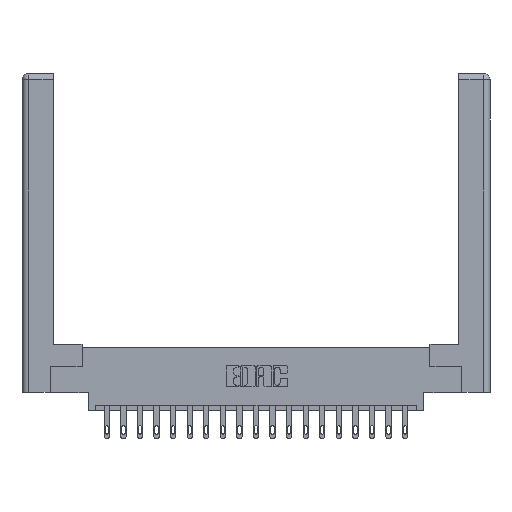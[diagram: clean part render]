
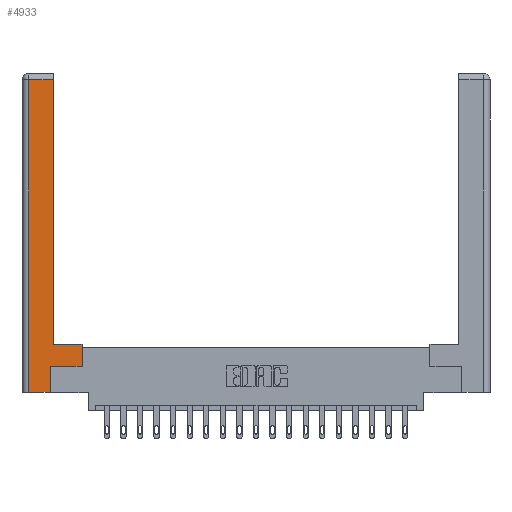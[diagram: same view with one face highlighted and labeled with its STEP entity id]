
A CAD part, top view. The second image highlights one B-rep face of the part: STEP entity #4933.
In plain terms, the highlighted planar face has unit normal (0, 0, 1).
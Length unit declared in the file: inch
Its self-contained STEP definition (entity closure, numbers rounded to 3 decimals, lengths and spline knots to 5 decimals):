
#195 = ORIENTED_EDGE ( 'NONE', *, *, #1138, .T. ) ;
#403 = VECTOR ( 'NONE', #12427, 39.37008 ) ;
#427 = LINE ( 'NONE', #4346, #16704 ) ;
#886 = LINE ( 'NONE', #3067, #8757 ) ;
#923 = DIRECTION ( 'NONE',  ( 1., 0., 0. ) ) ;
#1138 = EDGE_CURVE ( 'NONE', #15980, #16227, #7756, .T. ) ;
#1324 = LINE ( 'NONE', #5678, #8692 ) ;
#1429 = CARTESIAN_POINT ( 'NONE',  ( 0.295, 0.45, 0. ) ) ;
#2410 = CARTESIAN_POINT ( 'NONE',  ( 0.295, 2.94, 0. ) ) ;
#2630 = DIRECTION ( 'NONE',  ( -1., 0., 0. ) ) ;
#2715 = VERTEX_POINT ( 'NONE', #19667 ) ;
#2999 = CARTESIAN_POINT ( 'NONE',  ( 0.565, 0.245, 0. ) ) ;
#3067 = CARTESIAN_POINT ( 'NONE',  ( 0.565, 0.45, 0. ) ) ;
#3170 = CARTESIAN_POINT ( 'NONE',  ( 0.265, 0.245, 0. ) ) ;
#3243 = ORIENTED_EDGE ( 'NONE', *, *, #6716, .T. ) ;
#3328 = VECTOR ( 'NONE', #16255, 39.37008 ) ;
#4346 = CARTESIAN_POINT ( 'NONE',  ( 0.295, 0.45, 0. ) ) ;
#4414 = CARTESIAN_POINT ( 'NONE',  ( 0.565, 0.245, 0. ) ) ;
#4787 = DIRECTION ( 'NONE',  ( 0., 1., 0. ) ) ;
#4933 = ADVANCED_FACE ( 'NONE', ( #6801 ), #9155, .F. ) ;
#5036 = VERTEX_POINT ( 'NONE', #4414 ) ;
#5079 = CARTESIAN_POINT ( 'NONE',  ( 0.0615, 2.94, 0. ) ) ;
#5248 = ORIENTED_EDGE ( 'NONE', *, *, #15515, .T. ) ;
#5678 = CARTESIAN_POINT ( 'NONE',  ( 0.265, 0., 0. ) ) ;
#5732 = CARTESIAN_POINT ( 'NONE',  ( 0.565, 0.45, 0. ) ) ;
#5932 = CARTESIAN_POINT ( 'NONE',  ( 0., 0., 0. ) ) ;
#6716 = EDGE_CURVE ( 'NONE', #18542, #18761, #1324, .T. ) ;
#6801 = FACE_OUTER_BOUND ( 'NONE', #7833, .T. ) ;
#7376 = AXIS2_PLACEMENT_3D ( 'NONE', #5932, #15376, #17198 ) ;
#7696 = EDGE_CURVE ( 'NONE', #18761, #2715, #8650, .T. ) ;
#7756 = LINE ( 'NONE', #5079, #3328 ) ;
#7793 = CARTESIAN_POINT ( 'NONE',  ( 0.295, 3., 0. ) ) ;
#7833 = EDGE_LOOP ( 'NONE', ( #8580, #195, #16267, #3243, #14640, #5248, #8973, #11511 ) ) ;
#7989 = CARTESIAN_POINT ( 'NONE',  ( 0.0615, 2.94, 0. ) ) ;
#8081 = EDGE_CURVE ( 'NONE', #9605, #15980, #14572, .T. ) ;
#8413 = CARTESIAN_POINT ( 'NONE',  ( 0.0615, 0., 0. ) ) ;
#8580 = ORIENTED_EDGE ( 'NONE', *, *, #8081, .T. ) ;
#8650 = LINE ( 'NONE', #3170, #10888 ) ;
#8692 = VECTOR ( 'NONE', #923, 39.37008 ) ;
#8757 = VECTOR ( 'NONE', #4787, 39.37008 ) ;
#8973 = ORIENTED_EDGE ( 'NONE', *, *, #15477, .T. ) ;
#9155 = PLANE ( 'NONE',  #7376 ) ;
#9169 = DIRECTION ( 'NONE',  ( 0., 1., 0. ) ) ;
#9605 = VERTEX_POINT ( 'NONE', #1429 ) ;
#10888 = VECTOR ( 'NONE', #14320, 39.37008 ) ;
#11367 = VECTOR ( 'NONE', #9169, 39.37008 ) ;
#11511 = ORIENTED_EDGE ( 'NONE', *, *, #18788, .T. ) ;
#12427 = DIRECTION ( 'NONE',  ( 1., 0., 0. ) ) ;
#13210 = VECTOR ( 'NONE', #19576, 39.37008 ) ;
#13271 = CARTESIAN_POINT ( 'NONE',  ( 0.0615, 0., 0. ) ) ;
#13737 = VERTEX_POINT ( 'NONE', #5732 ) ;
#14320 = DIRECTION ( 'NONE',  ( 0., 1., 0. ) ) ;
#14448 = LINE ( 'NONE', #2999, #403 ) ;
#14572 = LINE ( 'NONE', #7793, #11367 ) ;
#14640 = ORIENTED_EDGE ( 'NONE', *, *, #7696, .T. ) ;
#15376 = DIRECTION ( 'NONE',  ( 0., 0., -1. ) ) ;
#15477 = EDGE_CURVE ( 'NONE', #5036, #13737, #886, .T. ) ;
#15515 = EDGE_CURVE ( 'NONE', #2715, #5036, #14448, .T. ) ;
#15980 = VERTEX_POINT ( 'NONE', #2410 ) ;
#16227 = VERTEX_POINT ( 'NONE', #7989 ) ;
#16255 = DIRECTION ( 'NONE',  ( -1., 0., 0. ) ) ;
#16267 = ORIENTED_EDGE ( 'NONE', *, *, #19137, .T. ) ;
#16704 = VECTOR ( 'NONE', #2630, 39.37008 ) ;
#17198 = DIRECTION ( 'NONE',  ( -1., 0., 0. ) ) ;
#17954 = LINE ( 'NONE', #13271, #13210 ) ;
#18542 = VERTEX_POINT ( 'NONE', #8413 ) ;
#18638 = CARTESIAN_POINT ( 'NONE',  ( 0.265, 0., 0. ) ) ;
#18761 = VERTEX_POINT ( 'NONE', #18638 ) ;
#18788 = EDGE_CURVE ( 'NONE', #13737, #9605, #427, .T. ) ;
#19137 = EDGE_CURVE ( 'NONE', #16227, #18542, #17954, .T. ) ;
#19576 = DIRECTION ( 'NONE',  ( 0., -1., 0. ) ) ;
#19667 = CARTESIAN_POINT ( 'NONE',  ( 0.265, 0.245, 0. ) ) ;
